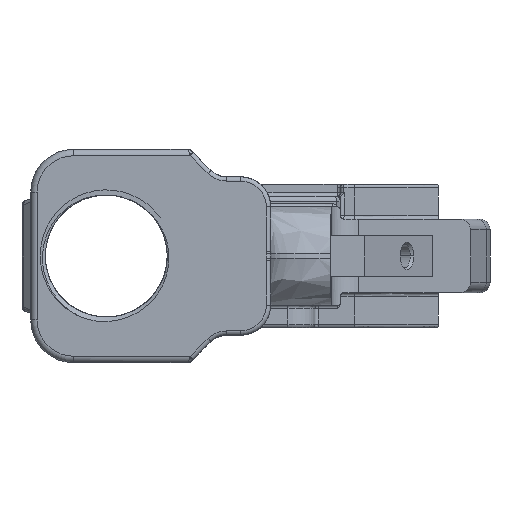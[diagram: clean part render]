
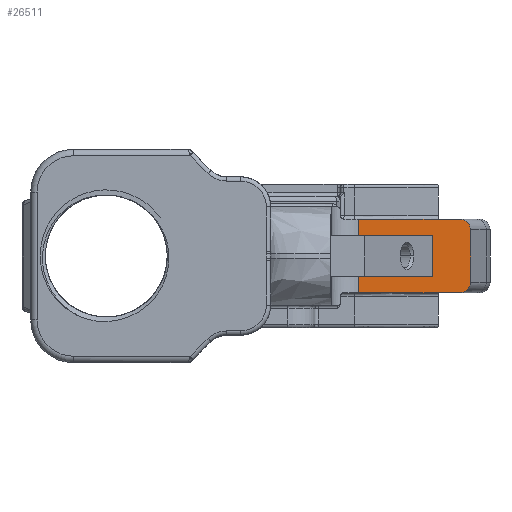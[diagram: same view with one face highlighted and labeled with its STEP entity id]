
A CAD part, left-side view. The second image highlights one B-rep face of the part: STEP entity #26511.
In plain terms, the highlighted planar face has unit normal (-1, 0, 0).
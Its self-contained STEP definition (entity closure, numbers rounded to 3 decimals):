
#1079 = ORIENTED_EDGE ( 'NONE', *, *, #33407, .F. ) ;
#1205 = CARTESIAN_POINT ( 'NONE',  ( -7.582, -69.52, -12.098 ) ) ;
#1207 = VECTOR ( 'NONE', #22223, 1000. ) ;
#1208 = LINE ( 'NONE', #5479, #8603 ) ;
#1395 = CARTESIAN_POINT ( 'NONE',  ( -7.582, -43.256, -13.151 ) ) ;
#1632 = VERTEX_POINT ( 'NONE', #27254 ) ;
#1849 = CARTESIAN_POINT ( 'NONE',  ( -7.582, -43.256, -9.264 ) ) ;
#1942 = VERTEX_POINT ( 'NONE', #24014 ) ;
#2315 = DIRECTION ( 'NONE',  ( 0., -1., 0. ) ) ;
#3088 = CARTESIAN_POINT ( 'NONE',  ( -7.582, -43.256, 0.261 ) ) ;
#3141 = VERTEX_POINT ( 'NONE', #21496 ) ;
#3350 = LINE ( 'NONE', #22347, #8972 ) ;
#3630 = LINE ( 'NONE', #6906, #11028 ) ;
#4537 = CARTESIAN_POINT ( 'NONE',  ( -7.582, -43.256, -12.636 ) ) ;
#5408 = VERTEX_POINT ( 'NONE', #15248 ) ;
#5479 = CARTESIAN_POINT ( 'NONE',  ( -7.582, -48.717, 0.261 ) ) ;
#5539 = EDGE_CURVE ( 'NONE', #20214, #26451, #33601, .T. ) ;
#5570 = CARTESIAN_POINT ( 'NONE',  ( -7.582, -56.388, -13.151 ) ) ;
#5734 = DIRECTION ( 'NONE',  ( 0., 0., -1. ) ) ;
#6578 = CARTESIAN_POINT ( 'NONE',  ( -7.582, -60.528, 0.261 ) ) ;
#6906 = CARTESIAN_POINT ( 'NONE',  ( -7.582, -43.256, 3.632 ) ) ;
#7816 = EDGE_CURVE ( 'NONE', #3141, #32586, #27520, .T. ) ;
#8285 = VECTOR ( 'NONE', #16939, 1000. ) ;
#8603 = VECTOR ( 'NONE', #22137, 1000. ) ;
#8972 = VECTOR ( 'NONE', #27915, 1000. ) ;
#9169 = LINE ( 'NONE', #22505, #8285 ) ;
#9471 = CARTESIAN_POINT ( 'NONE',  ( -7.582, -66.867, -13.151 ) ) ;
#9923 = LINE ( 'NONE', #19346, #17332 ) ;
#10167 = EDGE_CURVE ( 'NONE', #24468, #1942, #3630, .T. ) ;
#10300 = LINE ( 'NONE', #35710, #25076 ) ;
#10758 = CARTESIAN_POINT ( 'NONE',  ( -7.582, -69.52, 1.607 ) ) ;
#11028 = VECTOR ( 'NONE', #23552, 1000. ) ;
#11731 =( BOUNDED_CURVE ( )  B_SPLINE_CURVE ( 3, ( #9471, #12267, #1205, #20634 ),
 .UNSPECIFIED., .F., .F. ) 
 B_SPLINE_CURVE_WITH_KNOTS ( ( 4, 4 ),
 ( 4.712, 6.283 ),
 .UNSPECIFIED. ) 
 CURVE ( )  GEOMETRIC_REPRESENTATION_ITEM ( )  RATIONAL_B_SPLINE_CURVE ( ( 1., 0.805, 0.805, 1. ) ) 
 REPRESENTATION_ITEM ( '' )  );
#12267 = CARTESIAN_POINT ( 'NONE',  ( -7.582, -68.421, -13.151 ) ) ;
#12867 = ORIENTED_EDGE ( 'NONE', *, *, #15763, .T. ) ;
#13196 = ORIENTED_EDGE ( 'NONE', *, *, #10167, .F. ) ;
#13557 = CARTESIAN_POINT ( 'NONE',  ( -7.582, -66.867, 4.147 ) ) ;
#15248 = CARTESIAN_POINT ( 'NONE',  ( -7.582, -69.52, -10.611 ) ) ;
#15763 = EDGE_CURVE ( 'NONE', #1632, #26451, #9169, .T. ) ;
#15943 = CARTESIAN_POINT ( 'NONE',  ( -7.582, -69.52, 0.261 ) ) ;
#16939 = DIRECTION ( 'NONE',  ( 0., 1., 0. ) ) ;
#17332 = VECTOR ( 'NONE', #5734, 1000. ) ;
#17365 = ORIENTED_EDGE ( 'NONE', *, *, #22097, .T. ) ;
#18127 = EDGE_CURVE ( 'NONE', #27949, #5408, #11731, .T. ) ;
#18439 = ORIENTED_EDGE ( 'NONE', *, *, #7816, .T. ) ;
#18734 = DIRECTION ( 'NONE',  ( 0., 1., 0. ) ) ;
#18754 = EDGE_CURVE ( 'NONE', #1942, #32586, #10300, .T. ) ;
#18841 = VECTOR ( 'NONE', #23985, 1000. ) ;
#19346 = CARTESIAN_POINT ( 'NONE',  ( -7.582, -69.52, 2.204 ) ) ;
#19974 = AXIS2_PLACEMENT_3D ( 'NONE', #15943, #35369, #18734 ) ;
#20214 = VERTEX_POINT ( 'NONE', #1395 ) ;
#20634 = CARTESIAN_POINT ( 'NONE',  ( -7.582, -69.52, -10.611 ) ) ;
#21267 = PLANE ( 'NONE',  #19974 ) ;
#21496 = CARTESIAN_POINT ( 'NONE',  ( -7.582, -69.52, 1.607 ) ) ;
#22097 = EDGE_CURVE ( 'NONE', #20214, #27949, #23365, .T. ) ;
#22137 = DIRECTION ( 'NONE',  ( 0., 1., 0. ) ) ;
#22223 = DIRECTION ( 'NONE',  ( 0., -1., 0. ) ) ;
#22347 = CARTESIAN_POINT ( 'NONE',  ( -7.582, -60.528, -76.479 ) ) ;
#22505 = CARTESIAN_POINT ( 'NONE',  ( -7.582, -48.717, -9.264 ) ) ;
#23365 = LINE ( 'NONE', #5570, #1207 ) ;
#23552 = DIRECTION ( 'NONE',  ( 0., 0., 1. ) ) ;
#23985 = DIRECTION ( 'NONE',  ( 0., 0., 1. ) ) ;
#24014 = CARTESIAN_POINT ( 'NONE',  ( -7.582, -43.256, 4.147 ) ) ;
#24468 = VERTEX_POINT ( 'NONE', #3088 ) ;
#25076 = VECTOR ( 'NONE', #2315, 1000. ) ;
#26451 = VERTEX_POINT ( 'NONE', #1849 ) ;
#26511 = ADVANCED_FACE ( 'NONE', ( #33941 ), #21267, .F. ) ;
#27254 = CARTESIAN_POINT ( 'NONE',  ( -7.582, -60.528, -9.264 ) ) ;
#27385 = CARTESIAN_POINT ( 'NONE',  ( -7.582, -69.52, 3.095 ) ) ;
#27403 = ORIENTED_EDGE ( 'NONE', *, *, #27535, .F. ) ;
#27520 =( BOUNDED_CURVE ( )  B_SPLINE_CURVE ( 3, ( #10758, #27385, #30152, #13557 ),
 .UNSPECIFIED., .F., .F. ) 
 B_SPLINE_CURVE_WITH_KNOTS ( ( 4, 4 ),
 ( 0., 1.571 ),
 .UNSPECIFIED. ) 
 CURVE ( )  GEOMETRIC_REPRESENTATION_ITEM ( )  RATIONAL_B_SPLINE_CURVE ( ( 1., 0.805, 0.805, 1. ) ) 
 REPRESENTATION_ITEM ( '' )  );
#27535 = EDGE_CURVE ( 'NONE', #3141, #5408, #9923, .T. ) ;
#27632 = VERTEX_POINT ( 'NONE', #6578 ) ;
#27915 = DIRECTION ( 'NONE',  ( 0., 0., 1. ) ) ;
#27949 = VERTEX_POINT ( 'NONE', #30710 ) ;
#29175 = ORIENTED_EDGE ( 'NONE', *, *, #18754, .F. ) ;
#29333 = EDGE_LOOP ( 'NONE', ( #27403, #18439, #29175, #13196, #33746, #1079, #12867, #33698, #17365, #29355 ) ) ;
#29355 = ORIENTED_EDGE ( 'NONE', *, *, #18127, .T. ) ;
#30152 = CARTESIAN_POINT ( 'NONE',  ( -7.582, -68.421, 4.147 ) ) ;
#30710 = CARTESIAN_POINT ( 'NONE',  ( -7.582, -66.867, -13.151 ) ) ;
#32461 = CARTESIAN_POINT ( 'NONE',  ( -7.582, -66.867, 4.147 ) ) ;
#32586 = VERTEX_POINT ( 'NONE', #32461 ) ;
#33407 = EDGE_CURVE ( 'NONE', #1632, #27632, #3350, .T. ) ;
#33601 = LINE ( 'NONE', #4537, #18841 ) ;
#33698 = ORIENTED_EDGE ( 'NONE', *, *, #5539, .F. ) ;
#33746 = ORIENTED_EDGE ( 'NONE', *, *, #35756, .F. ) ;
#33941 = FACE_OUTER_BOUND ( 'NONE', #29333, .T. ) ;
#35369 = DIRECTION ( 'NONE',  ( 1., 0., 0. ) ) ;
#35710 = CARTESIAN_POINT ( 'NONE',  ( -7.582, -56.388, 4.147 ) ) ;
#35756 = EDGE_CURVE ( 'NONE', #27632, #24468, #1208, .T. ) ;
